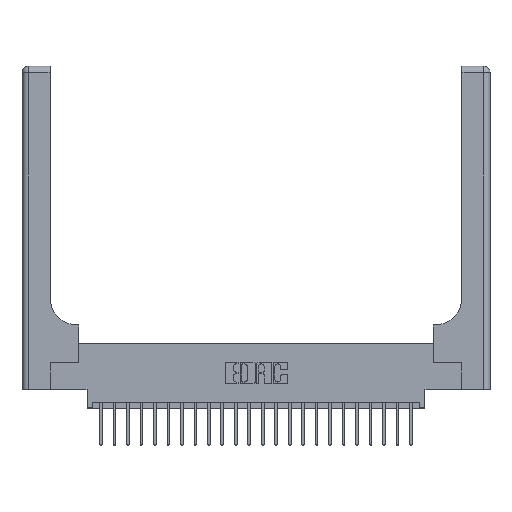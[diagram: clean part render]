
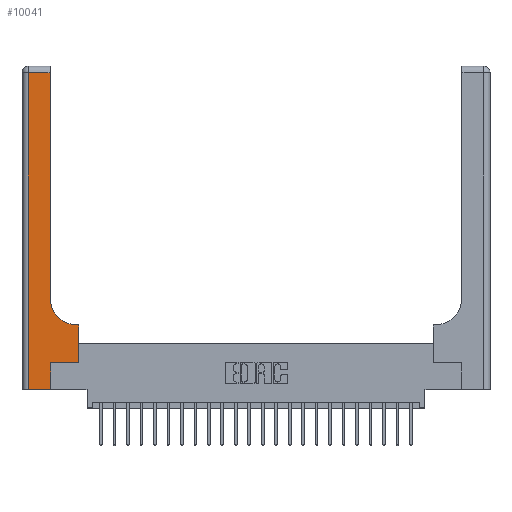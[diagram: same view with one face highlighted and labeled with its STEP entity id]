
A CAD part, top view. The second image highlights one B-rep face of the part: STEP entity #10041.
In plain terms, the highlighted planar face has unit normal (0, 0, 1).
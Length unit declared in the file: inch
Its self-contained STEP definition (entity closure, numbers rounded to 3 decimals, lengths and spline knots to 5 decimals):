
#569 = EDGE_CURVE ( 'NONE', #7674, #15387, #21130, .T. ) ;
#662 = CARTESIAN_POINT ( 'NONE',  ( 0.26, 2.94, 0.37 ) ) ;
#1537 = CARTESIAN_POINT ( 'NONE',  ( 0.26, 3., 0.37 ) ) ;
#1705 = CARTESIAN_POINT ( 'NONE',  ( 0.26, 0.6, 0.37 ) ) ;
#1792 = VECTOR ( 'NONE', #4888, 39.37008 ) ;
#2538 = DIRECTION ( 'NONE',  ( 0., 0., -1. ) ) ;
#2706 = EDGE_CURVE ( 'NONE', #22049, #7674, #8376, .T. ) ;
#2937 = ORIENTED_EDGE ( 'NONE', *, *, #10000, .T. ) ;
#3027 = CARTESIAN_POINT ( 'NONE',  ( 0., 2.94, 0.37 ) ) ;
#3125 = DIRECTION ( 'NONE',  ( 1., 0., 0. ) ) ;
#3628 = DIRECTION ( 'NONE',  ( 0., 1., 0. ) ) ;
#3682 = LINE ( 'NONE', #14479, #22316 ) ;
#4519 = ORIENTED_EDGE ( 'NONE', *, *, #5478, .T. ) ;
#4614 = CARTESIAN_POINT ( 'NONE',  ( 0.26, 0.85, 0.37 ) ) ;
#4888 = DIRECTION ( 'NONE',  ( -1., 0., 0. ) ) ;
#4961 = CARTESIAN_POINT ( 'NONE',  ( 0., 3., 0.37 ) ) ;
#5364 = DIRECTION ( 'NONE',  ( -1., 0., 0. ) ) ;
#5478 = EDGE_CURVE ( 'NONE', #19388, #22049, #3682, .T. ) ;
#5804 = CARTESIAN_POINT ( 'NONE',  ( 0.51, 0.6, 0.37 ) ) ;
#5813 = EDGE_CURVE ( 'NONE', #8788, #13328, #16098, .T. ) ;
#6315 = LINE ( 'NONE', #21580, #20152 ) ;
#6358 = CARTESIAN_POINT ( 'NONE',  ( 0.06, 3., 0.37 ) ) ;
#6512 = VECTOR ( 'NONE', #12381, 39.37008 ) ;
#6720 = CARTESIAN_POINT ( 'NONE',  ( 0.265, 0.25, 0.37 ) ) ;
#6891 = AXIS2_PLACEMENT_3D ( 'NONE', #4961, #22995, #12226 ) ;
#7376 = ORIENTED_EDGE ( 'NONE', *, *, #2706, .T. ) ;
#7674 = VERTEX_POINT ( 'NONE', #14762 ) ;
#7717 = LINE ( 'NONE', #1705, #10813 ) ;
#8163 = DIRECTION ( 'NONE',  ( 0., -1., 0. ) ) ;
#8376 = LINE ( 'NONE', #6720, #17404 ) ;
#8424 = CARTESIAN_POINT ( 'NONE',  ( 0.265, 0.25, 0.37 ) ) ;
#8788 = VERTEX_POINT ( 'NONE', #4614 ) ;
#8952 = CARTESIAN_POINT ( 'NONE',  ( 0.265, 0., 0.37 ) ) ;
#8971 = DIRECTION ( 'NONE',  ( 1., 0., 0. ) ) ;
#8991 = ORIENTED_EDGE ( 'NONE', *, *, #19083, .T. ) ;
#9192 = DIRECTION ( 'NONE',  ( 0., 1., 0. ) ) ;
#9893 = CARTESIAN_POINT ( 'NONE',  ( 0.06, 0., 0.37 ) ) ;
#10000 = EDGE_CURVE ( 'NONE', #13328, #14615, #16783, .T. ) ;
#10041 = ADVANCED_FACE ( 'NONE', ( #11426 ), #10405, .F. ) ;
#10151 = ORIENTED_EDGE ( 'NONE', *, *, #11725, .T. ) ;
#10405 = PLANE ( 'NONE',  #6891 ) ;
#10780 = EDGE_CURVE ( 'NONE', #11044, #19388, #6315, .T. ) ;
#10813 = VECTOR ( 'NONE', #5364, 39.37008 ) ;
#10870 = ORIENTED_EDGE ( 'NONE', *, *, #23308, .T. ) ;
#11044 = VERTEX_POINT ( 'NONE', #9893 ) ;
#11292 = EDGE_LOOP ( 'NONE', ( #14505, #2937, #8991, #21650, #4519, #7376, #14726, #10151, #10870 ) ) ;
#11426 = FACE_OUTER_BOUND ( 'NONE', #11292, .T. ) ;
#11725 = EDGE_CURVE ( 'NONE', #15387, #20839, #7717, .T. ) ;
#12226 = DIRECTION ( 'NONE',  ( -1., 0., 0. ) ) ;
#12381 = DIRECTION ( 'NONE',  ( 0., 1., 0. ) ) ;
#12680 = VECTOR ( 'NONE', #8163, 39.37008 ) ;
#12798 = CIRCLE ( 'NONE', #19103, 0.25 ) ;
#13328 = VERTEX_POINT ( 'NONE', #662 ) ;
#13386 = CARTESIAN_POINT ( 'NONE',  ( 0.51, 0.85, 0.37 ) ) ;
#14479 = CARTESIAN_POINT ( 'NONE',  ( 0.265, 0., 0.37 ) ) ;
#14505 = ORIENTED_EDGE ( 'NONE', *, *, #5813, .T. ) ;
#14615 = VERTEX_POINT ( 'NONE', #19832 ) ;
#14726 = ORIENTED_EDGE ( 'NONE', *, *, #569, .T. ) ;
#14762 = CARTESIAN_POINT ( 'NONE',  ( 0.528, 0.25, 0.37 ) ) ;
#15214 = DIRECTION ( 'NONE',  ( 1., 0., 0. ) ) ;
#15387 = VERTEX_POINT ( 'NONE', #17274 ) ;
#16098 = LINE ( 'NONE', #1537, #6512 ) ;
#16783 = LINE ( 'NONE', #3027, #1792 ) ;
#17274 = CARTESIAN_POINT ( 'NONE',  ( 0.528, 0.6, 0.37 ) ) ;
#17404 = VECTOR ( 'NONE', #3125, 39.37008 ) ;
#17467 = VECTOR ( 'NONE', #9192, 39.37008 ) ;
#19083 = EDGE_CURVE ( 'NONE', #14615, #11044, #22801, .T. ) ;
#19103 = AXIS2_PLACEMENT_3D ( 'NONE', #13386, #2538, #15214 ) ;
#19388 = VERTEX_POINT ( 'NONE', #8952 ) ;
#19832 = CARTESIAN_POINT ( 'NONE',  ( 0.06, 2.94, 0.37 ) ) ;
#20152 = VECTOR ( 'NONE', #8971, 39.37008 ) ;
#20839 = VERTEX_POINT ( 'NONE', #5804 ) ;
#21130 = LINE ( 'NONE', #21723, #17467 ) ;
#21580 = CARTESIAN_POINT ( 'NONE',  ( 0., 0., 0.37 ) ) ;
#21650 = ORIENTED_EDGE ( 'NONE', *, *, #10780, .T. ) ;
#21723 = CARTESIAN_POINT ( 'NONE',  ( 0.528, 0.25, 0.37 ) ) ;
#22049 = VERTEX_POINT ( 'NONE', #8424 ) ;
#22316 = VECTOR ( 'NONE', #3628, 39.37008 ) ;
#22801 = LINE ( 'NONE', #6358, #12680 ) ;
#22995 = DIRECTION ( 'NONE',  ( 0., 0., -1. ) ) ;
#23308 = EDGE_CURVE ( 'NONE', #20839, #8788, #12798, .T. ) ;
